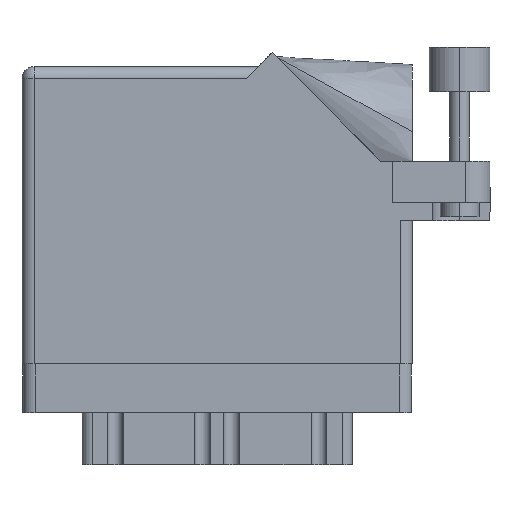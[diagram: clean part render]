
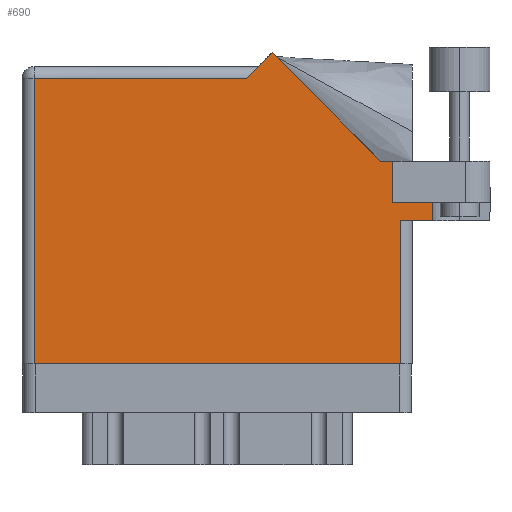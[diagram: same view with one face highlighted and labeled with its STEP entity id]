
A CAD part, front view. The second image highlights one B-rep face of the part: STEP entity #690.
In plain terms, the highlighted face is planar.
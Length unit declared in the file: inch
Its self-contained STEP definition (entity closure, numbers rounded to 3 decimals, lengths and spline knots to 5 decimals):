
#281 = VECTOR ( 'NONE', #26114, 39.37008 ) ;
#690 = ADVANCED_FACE ( 'NONE', ( #18332 ), #18162, .F. ) ;
#782 = VECTOR ( 'NONE', #15896, 39.37008 ) ;
#1116 = VERTEX_POINT ( 'NONE', #6886 ) ;
#1651 = VECTOR ( 'NONE', #32039, 39.37008 ) ;
#2458 = EDGE_CURVE ( 'NONE', #21838, #22198, #31976, .T. ) ;
#2687 = VERTEX_POINT ( 'NONE', #14516 ) ;
#2760 = VECTOR ( 'NONE', #13781, 39.37008 ) ;
#2923 = DIRECTION ( 'NONE',  ( -1., 0., 0. ) ) ;
#4110 = LINE ( 'NONE', #22147, #19615 ) ;
#5050 = DIRECTION ( 'NONE',  ( 0., -1., 0. ) ) ;
#5152 = EDGE_CURVE ( 'NONE', #19998, #28659, #34985, .T. ) ;
#5217 = CARTESIAN_POINT ( 'NONE',  ( 2.41, 1.044, 0. ) ) ;
#5600 = EDGE_LOOP ( 'NONE', ( #21120, #21603, #9210, #35080, #19473, #7214, #30453, #22027, #5634, #31632, #10099 ) ) ;
#5634 = ORIENTED_EDGE ( 'NONE', *, *, #28507, .T. ) ;
#6873 = CARTESIAN_POINT ( 'NONE',  ( 1.155, 1.468, 0. ) ) ;
#6886 = CARTESIAN_POINT ( 'NONE',  ( 2.1115, 0.831, 0. ) ) ;
#7214 = ORIENTED_EDGE ( 'NONE', *, *, #17260, .T. ) ;
#7480 = CARTESIAN_POINT ( 'NONE',  ( 1.91, 0.831, 0. ) ) ;
#7695 = CARTESIAN_POINT ( 'NONE',  ( 0.062, 0., 0. ) ) ;
#8435 = CARTESIAN_POINT ( 'NONE',  ( 1.91, 0.831, 0. ) ) ;
#9073 = CARTESIAN_POINT ( 'NONE',  ( 2.01, 0.737, 0. ) ) ;
#9108 = CARTESIAN_POINT ( 'NONE',  ( 1.91, 1.044, 0. ) ) ;
#9121 = DIRECTION ( 'NONE',  ( 1., 0., 0. ) ) ;
#9210 = ORIENTED_EDGE ( 'NONE', *, *, #2458, .T. ) ;
#9362 = VECTOR ( 'NONE', #25892, 39.37008 ) ;
#9481 = CARTESIAN_POINT ( 'NONE',  ( 0., 0., 0. ) ) ;
#9745 = VERTEX_POINT ( 'NONE', #18490 ) ;
#9955 = CARTESIAN_POINT ( 'NONE',  ( 0., 1.53, 0. ) ) ;
#10099 = ORIENTED_EDGE ( 'NONE', *, *, #16589, .T. ) ;
#10376 = LINE ( 'NONE', #7695, #18062 ) ;
#11988 = LINE ( 'NONE', #12352, #9362 ) ;
#12352 = CARTESIAN_POINT ( 'NONE',  ( 1.217, 1.53, 0. ) ) ;
#12478 = LINE ( 'NONE', #25671, #12630 ) ;
#12621 = DIRECTION ( 'NONE',  ( 0., 0., -1. ) ) ;
#12630 = VECTOR ( 'NONE', #23177, 39.37008 ) ;
#13781 = DIRECTION ( 'NONE',  ( 0., 1., 0. ) ) ;
#13951 = EDGE_CURVE ( 'NONE', #28030, #2687, #4110, .T. ) ;
#14193 = VERTEX_POINT ( 'NONE', #26700 ) ;
#14516 = CARTESIAN_POINT ( 'NONE',  ( 0.062, 1.468, 0. ) ) ;
#15896 = DIRECTION ( 'NONE',  ( -1., 0., 0. ) ) ;
#16417 = LINE ( 'NONE', #5217, #782 ) ;
#16589 = EDGE_CURVE ( 'NONE', #2687, #14193, #10376, .T. ) ;
#17198 = CARTESIAN_POINT ( 'NONE',  ( 1.948, 0.737, 0. ) ) ;
#17260 = EDGE_CURVE ( 'NONE', #18187, #29507, #24325, .T. ) ;
#18022 = AXIS2_PLACEMENT_3D ( 'NONE', #9955, #12621, #26691 ) ;
#18062 = VECTOR ( 'NONE', #5050, 39.37008 ) ;
#18162 = PLANE ( 'NONE',  #18022 ) ;
#18187 = VERTEX_POINT ( 'NONE', #7480 ) ;
#18276 = LINE ( 'NONE', #31786, #281 ) ;
#18332 = FACE_OUTER_BOUND ( 'NONE', #5600, .T. ) ;
#18385 = VECTOR ( 'NONE', #9121, 39.37008 ) ;
#18490 = CARTESIAN_POINT ( 'NONE',  ( 1.948, 0., 0. ) ) ;
#18807 = CARTESIAN_POINT ( 'NONE',  ( 1.84442, 1.044, 0. ) ) ;
#18978 = DIRECTION ( 'NONE',  ( -0.707, 0.707, 0. ) ) ;
#19204 = CARTESIAN_POINT ( 'NONE',  ( 1.84442, 1.044, 0. ) ) ;
#19372 = EDGE_CURVE ( 'NONE', #1116, #22198, #26552, .T. ) ;
#19473 = ORIENTED_EDGE ( 'NONE', *, *, #28024, .F. ) ;
#19615 = VECTOR ( 'NONE', #2923, 39.37008 ) ;
#19998 = VERTEX_POINT ( 'NONE', #19204 ) ;
#20806 = VECTOR ( 'NONE', #23292, 39.37008 ) ;
#21120 = ORIENTED_EDGE ( 'NONE', *, *, #25400, .T. ) ;
#21603 = ORIENTED_EDGE ( 'NONE', *, *, #24170, .T. ) ;
#21838 = VERTEX_POINT ( 'NONE', #17198 ) ;
#22027 = ORIENTED_EDGE ( 'NONE', *, *, #5152, .T. ) ;
#22147 = CARTESIAN_POINT ( 'NONE',  ( 0., 1.468, 0. ) ) ;
#22198 = VERTEX_POINT ( 'NONE', #30001 ) ;
#23177 = DIRECTION ( 'NONE',  ( 0., 1., 0. ) ) ;
#23292 = DIRECTION ( 'NONE',  ( 1., 0., 0. ) ) ;
#24063 = CARTESIAN_POINT ( 'NONE',  ( 2.1115, 1.16177, 0. ) ) ;
#24170 = EDGE_CURVE ( 'NONE', #9745, #21838, #12478, .T. ) ;
#24325 = LINE ( 'NONE', #8435, #2760 ) ;
#25400 = EDGE_CURVE ( 'NONE', #14193, #9745, #30505, .T. ) ;
#25671 = CARTESIAN_POINT ( 'NONE',  ( 1.948, 0.737, 0. ) ) ;
#25706 = EDGE_CURVE ( 'NONE', #29507, #19998, #16417, .T. ) ;
#25892 = DIRECTION ( 'NONE',  ( -0.707, -0.707, 0. ) ) ;
#26114 = DIRECTION ( 'NONE',  ( 1., 0., 0. ) ) ;
#26552 = LINE ( 'NONE', #24063, #1651 ) ;
#26691 = DIRECTION ( 'NONE',  ( -1., 0., 0. ) ) ;
#26700 = CARTESIAN_POINT ( 'NONE',  ( 0.062, 0., 0. ) ) ;
#28024 = EDGE_CURVE ( 'NONE', #18187, #1116, #18276, .T. ) ;
#28030 = VERTEX_POINT ( 'NONE', #6873 ) ;
#28507 = EDGE_CURVE ( 'NONE', #28659, #28030, #11988, .T. ) ;
#28659 = VERTEX_POINT ( 'NONE', #33100 ) ;
#29460 = VECTOR ( 'NONE', #18978, 39.37008 ) ;
#29507 = VERTEX_POINT ( 'NONE', #9108 ) ;
#30001 = CARTESIAN_POINT ( 'NONE',  ( 2.1115, 0.737, 0. ) ) ;
#30453 = ORIENTED_EDGE ( 'NONE', *, *, #25706, .T. ) ;
#30505 = LINE ( 'NONE', #9481, #18385 ) ;
#31632 = ORIENTED_EDGE ( 'NONE', *, *, #13951, .T. ) ;
#31786 = CARTESIAN_POINT ( 'NONE',  ( 1.91, 0.831, 0. ) ) ;
#31976 = LINE ( 'NONE', #9073, #20806 ) ;
#32039 = DIRECTION ( 'NONE',  ( 0., -1., 0. ) ) ;
#33100 = CARTESIAN_POINT ( 'NONE',  ( 1.28771, 1.60071, 0. ) ) ;
#34985 = LINE ( 'NONE', #18807, #29460 ) ;
#35080 = ORIENTED_EDGE ( 'NONE', *, *, #19372, .F. ) ;
